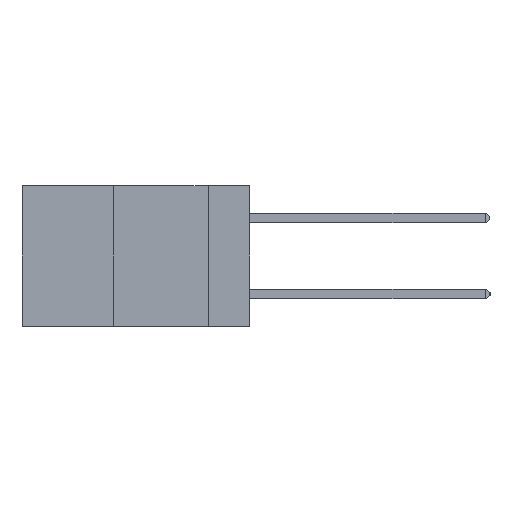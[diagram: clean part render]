
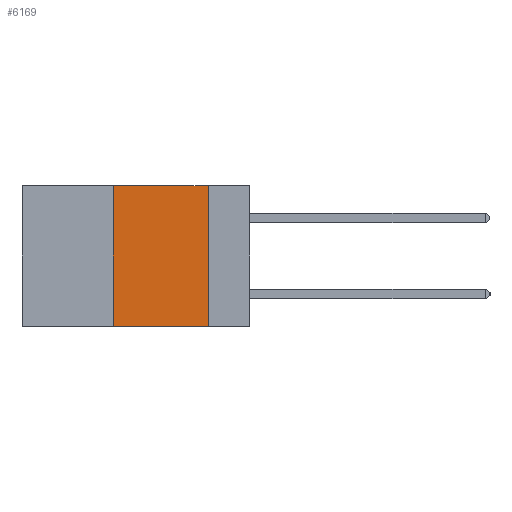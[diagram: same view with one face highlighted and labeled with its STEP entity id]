
A CAD part, left-side view. The second image highlights one B-rep face of the part: STEP entity #6169.
In plain terms, the highlighted planar face has unit normal (-1, 0, 0).
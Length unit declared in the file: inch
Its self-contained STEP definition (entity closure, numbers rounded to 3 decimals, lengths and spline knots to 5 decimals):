
#341 = CARTESIAN_POINT ( 'NONE',  ( 0., 0.36, 0. ) ) ;
#785 = DIRECTION ( 'NONE',  ( 0., 0., -1. ) ) ;
#1008 = ORIENTED_EDGE ( 'NONE', *, *, #13472, .F. ) ;
#1129 = CARTESIAN_POINT ( 'NONE',  ( 0., 0.11, 0. ) ) ;
#1958 = DIRECTION ( 'NONE',  ( 0., 0., -1. ) ) ;
#2314 = VERTEX_POINT ( 'NONE', #5954 ) ;
#2954 = DIRECTION ( 'NONE',  ( 0., 0., 1. ) ) ;
#3741 = EDGE_CURVE ( 'NONE', #13359, #6623, #11319, .T. ) ;
#5083 = VECTOR ( 'NONE', #785, 39.37008 ) ;
#5406 = ORIENTED_EDGE ( 'NONE', *, *, #3741, .F. ) ;
#5567 = EDGE_CURVE ( 'NONE', #10236, #6623, #10833, .T. ) ;
#5954 = CARTESIAN_POINT ( 'NONE',  ( 0., 0.36, 0. ) ) ;
#6098 = CARTESIAN_POINT ( 'NONE',  ( 0., 0.11, 0. ) ) ;
#6169 = ADVANCED_FACE ( 'NONE', ( #8076 ), #16286, .F. ) ;
#6310 = VECTOR ( 'NONE', #15496, 39.37008 ) ;
#6623 = VERTEX_POINT ( 'NONE', #6638 ) ;
#6638 = CARTESIAN_POINT ( 'NONE',  ( 0., 0.11, -0.37 ) ) ;
#7065 = ORIENTED_EDGE ( 'NONE', *, *, #14382, .F. ) ;
#7896 = EDGE_LOOP ( 'NONE', ( #5406, #1008, #7065, #15704 ) ) ;
#8076 = FACE_OUTER_BOUND ( 'NONE', #7896, .T. ) ;
#8471 = CARTESIAN_POINT ( 'NONE',  ( 0., 0.6, 0. ) ) ;
#8549 = DIRECTION ( 'NONE',  ( 0., -1., 0. ) ) ;
#9819 = DIRECTION ( 'NONE',  ( 1., 0., 0. ) ) ;
#9872 = LINE ( 'NONE', #14216, #6310 ) ;
#10236 = VERTEX_POINT ( 'NONE', #14751 ) ;
#10302 = AXIS2_PLACEMENT_3D ( 'NONE', #8471, #9819, #1958 ) ;
#10417 = VECTOR ( 'NONE', #8549, 39.37008 ) ;
#10833 = LINE ( 'NONE', #12577, #10417 ) ;
#11319 = LINE ( 'NONE', #1129, #5083 ) ;
#12577 = CARTESIAN_POINT ( 'NONE',  ( 0., 0.6, -0.37 ) ) ;
#13148 = LINE ( 'NONE', #341, #16159 ) ;
#13359 = VERTEX_POINT ( 'NONE', #6098 ) ;
#13472 = EDGE_CURVE ( 'NONE', #2314, #13359, #9872, .T. ) ;
#14216 = CARTESIAN_POINT ( 'NONE',  ( 0., 0.6, 0. ) ) ;
#14382 = EDGE_CURVE ( 'NONE', #10236, #2314, #13148, .T. ) ;
#14751 = CARTESIAN_POINT ( 'NONE',  ( 0., 0.36, -0.37 ) ) ;
#15496 = DIRECTION ( 'NONE',  ( 0., -1., 0. ) ) ;
#15704 = ORIENTED_EDGE ( 'NONE', *, *, #5567, .T. ) ;
#16159 = VECTOR ( 'NONE', #2954, 39.37008 ) ;
#16286 = PLANE ( 'NONE',  #10302 ) ;
